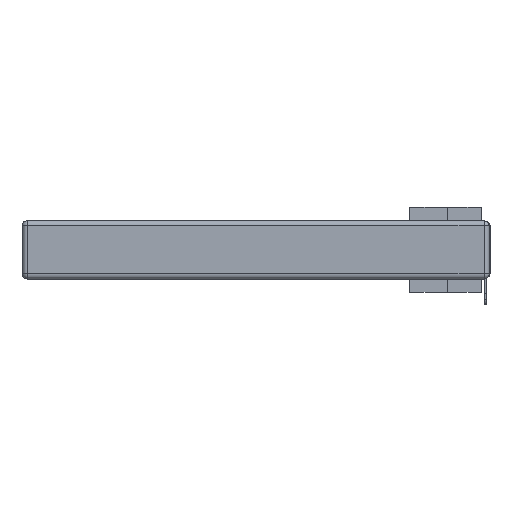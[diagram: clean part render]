
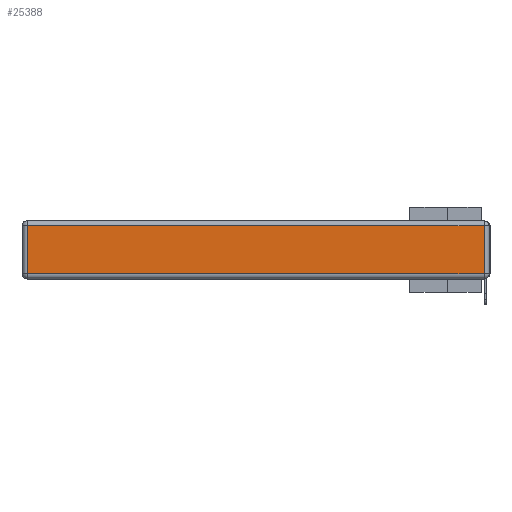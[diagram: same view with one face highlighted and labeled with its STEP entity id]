
A CAD part, left-side view. The second image highlights one B-rep face of the part: STEP entity #25388.
In plain terms, the highlighted planar face has unit normal (-1, 0, 0).
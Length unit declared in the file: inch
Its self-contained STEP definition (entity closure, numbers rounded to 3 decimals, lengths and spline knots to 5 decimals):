
#600 = FACE_OUTER_BOUND ( 'NONE', #17559, .T. ) ;
#1481 = VERTEX_POINT ( 'NONE', #5063 ) ;
#2621 = ORIENTED_EDGE ( 'NONE', *, *, #32128, .T. ) ;
#3677 = CARTESIAN_POINT ( 'NONE',  ( 0., 2.75, -0.03 ) ) ;
#3900 = CARTESIAN_POINT ( 'NONE',  ( 0., 2.72, -0.03 ) ) ;
#4068 = VECTOR ( 'NONE', #21568, 39.37008 ) ;
#4700 = CARTESIAN_POINT ( 'NONE',  ( 0., 2.72, -0.343 ) ) ;
#5063 = CARTESIAN_POINT ( 'NONE',  ( 0., 0.03, -0.313 ) ) ;
#5885 = VERTEX_POINT ( 'NONE', #3900 ) ;
#7533 = EDGE_CURVE ( 'NONE', #29165, #1481, #15771, .T. ) ;
#7733 = CARTESIAN_POINT ( 'NONE',  ( 0., 0.03, -0.343 ) ) ;
#8333 = DIRECTION ( 'NONE',  ( -1., 0., 0. ) ) ;
#10524 = ORIENTED_EDGE ( 'NONE', *, *, #15198, .T. ) ;
#10558 = CARTESIAN_POINT ( 'NONE',  ( 0., 2.72, -0.313 ) ) ;
#10825 = PLANE ( 'NONE',  #31991 ) ;
#12241 = VERTEX_POINT ( 'NONE', #18197 ) ;
#12244 = DIRECTION ( 'NONE',  ( 0., 0., 1. ) ) ;
#14723 = DIRECTION ( 'NONE',  ( 0., 0., -1. ) ) ;
#15198 = EDGE_CURVE ( 'NONE', #1481, #12241, #30483, .T. ) ;
#15450 = ORIENTED_EDGE ( 'NONE', *, *, #7533, .T. ) ;
#15771 = LINE ( 'NONE', #28990, #19538 ) ;
#17559 = EDGE_LOOP ( 'NONE', ( #15450, #10524, #2621, #18743 ) ) ;
#18197 = CARTESIAN_POINT ( 'NONE',  ( 0., 0.03, -0.03 ) ) ;
#18743 = ORIENTED_EDGE ( 'NONE', *, *, #26497, .T. ) ;
#19538 = VECTOR ( 'NONE', #25988, 39.37008 ) ;
#19756 = LINE ( 'NONE', #4700, #23574 ) ;
#20902 = LINE ( 'NONE', #3677, #4068 ) ;
#21568 = DIRECTION ( 'NONE',  ( 0., 1., 0. ) ) ;
#23574 = VECTOR ( 'NONE', #14723, 39.37008 ) ;
#24370 = DIRECTION ( 'NONE',  ( 0., 0., 1. ) ) ;
#25074 = VECTOR ( 'NONE', #12244, 39.37008 ) ;
#25388 = ADVANCED_FACE ( 'NONE', ( #600 ), #10825, .T. ) ;
#25988 = DIRECTION ( 'NONE',  ( 0., -1., 0. ) ) ;
#26497 = EDGE_CURVE ( 'NONE', #5885, #29165, #19756, .T. ) ;
#28990 = CARTESIAN_POINT ( 'NONE',  ( 0., 0., -0.313 ) ) ;
#29165 = VERTEX_POINT ( 'NONE', #10558 ) ;
#30483 = LINE ( 'NONE', #7733, #25074 ) ;
#31248 = CARTESIAN_POINT ( 'NONE',  ( 0., 0., -0.343 ) ) ;
#31991 = AXIS2_PLACEMENT_3D ( 'NONE', #31248, #8333, #24370 ) ;
#32128 = EDGE_CURVE ( 'NONE', #12241, #5885, #20902, .T. ) ;
